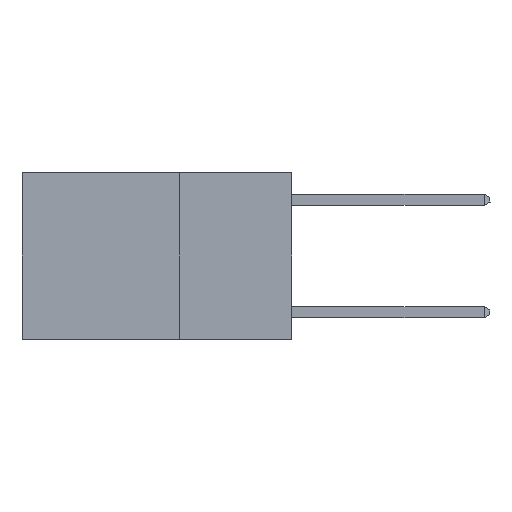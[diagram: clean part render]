
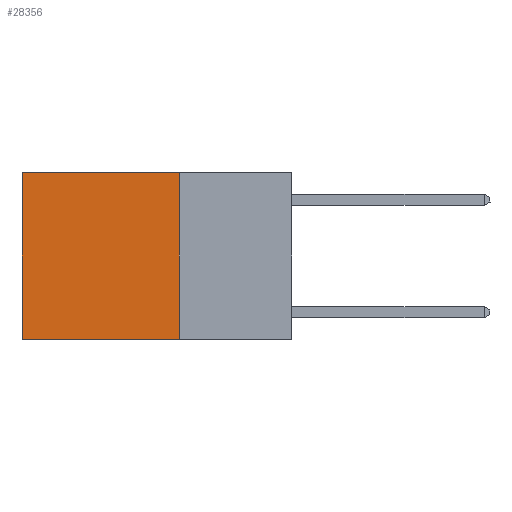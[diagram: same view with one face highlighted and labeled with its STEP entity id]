
A CAD part, left-side view. The second image highlights one B-rep face of the part: STEP entity #28356.
In plain terms, the highlighted planar face has unit normal (-1, 0, 0).
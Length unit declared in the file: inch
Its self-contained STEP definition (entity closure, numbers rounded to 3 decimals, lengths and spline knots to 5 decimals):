
#436 = ORIENTED_EDGE ( 'NONE', *, *, #25866, .F. ) ;
#1044 = EDGE_CURVE ( 'NONE', #30315, #28820, #15921, .T. ) ;
#1118 = EDGE_LOOP ( 'NONE', ( #12069, #24464, #436, #7614 ) ) ;
#1887 = VECTOR ( 'NONE', #7382, 39.37008 ) ;
#3657 = CARTESIAN_POINT ( 'NONE',  ( 0.2625, 0.25, 0. ) ) ;
#4653 = FACE_OUTER_BOUND ( 'NONE', #1118, .T. ) ;
#7382 = DIRECTION ( 'NONE',  ( 0., 0., -1. ) ) ;
#7614 = ORIENTED_EDGE ( 'NONE', *, *, #1044, .T. ) ;
#8437 = EDGE_CURVE ( 'NONE', #21916, #24277, #18394, .T. ) ;
#8500 = DIRECTION ( 'NONE',  ( 0., 0., -1. ) ) ;
#10996 = DIRECTION ( 'NONE',  ( 0., 0., -1. ) ) ;
#11174 = CARTESIAN_POINT ( 'NONE',  ( 0.2625, 0.25, 0. ) ) ;
#12069 = ORIENTED_EDGE ( 'NONE', *, *, #28168, .T. ) ;
#12128 = CARTESIAN_POINT ( 'NONE',  ( 0.2625, 0.25, 0. ) ) ;
#13156 = CARTESIAN_POINT ( 'NONE',  ( 0.2625, 0.25, 0. ) ) ;
#14763 = LINE ( 'NONE', #12128, #1887 ) ;
#15921 = LINE ( 'NONE', #13156, #25178 ) ;
#15989 = CARTESIAN_POINT ( 'NONE',  ( 0.2625, 0.25, -0.37 ) ) ;
#16363 = CARTESIAN_POINT ( 'NONE',  ( 0.2625, 0.6, 0. ) ) ;
#16793 = LINE ( 'NONE', #20594, #21992 ) ;
#17504 = DIRECTION ( 'NONE',  ( 0., 1., 0. ) ) ;
#18394 = LINE ( 'NONE', #15989, #28716 ) ;
#20372 = DIRECTION ( 'NONE',  ( 1., 0., 0. ) ) ;
#20594 = CARTESIAN_POINT ( 'NONE',  ( 0.2625, 0.6, 0. ) ) ;
#20743 = DIRECTION ( 'NONE',  ( 0., 1., 0. ) ) ;
#21916 = VERTEX_POINT ( 'NONE', #26448 ) ;
#21992 = VECTOR ( 'NONE', #10996, 39.37008 ) ;
#22209 = AXIS2_PLACEMENT_3D ( 'NONE', #3657, #20372, #8500 ) ;
#24277 = VERTEX_POINT ( 'NONE', #26246 ) ;
#24341 = PLANE ( 'NONE',  #22209 ) ;
#24464 = ORIENTED_EDGE ( 'NONE', *, *, #8437, .F. ) ;
#25178 = VECTOR ( 'NONE', #17504, 39.37008 ) ;
#25866 = EDGE_CURVE ( 'NONE', #30315, #21916, #14763, .T. ) ;
#26246 = CARTESIAN_POINT ( 'NONE',  ( 0.2625, 0.6, -0.37 ) ) ;
#26448 = CARTESIAN_POINT ( 'NONE',  ( 0.2625, 0.25, -0.37 ) ) ;
#28168 = EDGE_CURVE ( 'NONE', #28820, #24277, #16793, .T. ) ;
#28356 = ADVANCED_FACE ( 'NONE', ( #4653 ), #24341, .F. ) ;
#28716 = VECTOR ( 'NONE', #20743, 39.37008 ) ;
#28820 = VERTEX_POINT ( 'NONE', #16363 ) ;
#30315 = VERTEX_POINT ( 'NONE', #11174 ) ;
